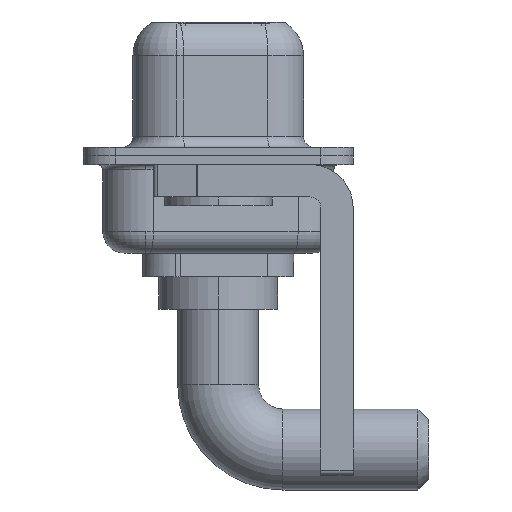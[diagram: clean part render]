
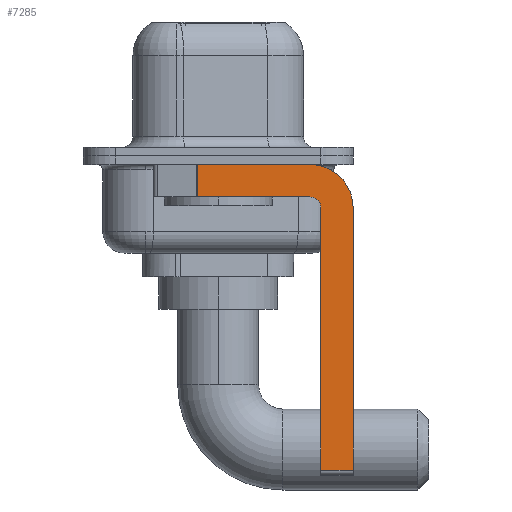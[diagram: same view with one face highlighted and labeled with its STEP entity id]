
A CAD part, left-side view. The second image highlights one B-rep face of the part: STEP entity #7285.
In plain terms, the highlighted planar face has unit normal (-1, 0, 0).
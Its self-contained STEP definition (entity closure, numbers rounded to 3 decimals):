
#55 = VERTEX_POINT ( 'NONE', #4018 ) ;
#355 = DIRECTION ( 'NONE',  ( 1., 0., 0. ) ) ;
#384 = VERTEX_POINT ( 'NONE', #9413 ) ;
#775 = LINE ( 'NONE', #13103, #7218 ) ;
#920 = ORIENTED_EDGE ( 'NONE', *, *, #1465, .F. ) ;
#1044 = CIRCLE ( 'NONE', #12889, 2. ) ;
#1110 = VECTOR ( 'NONE', #9115, 1000. ) ;
#1119 = EDGE_LOOP ( 'NONE', ( #3318, #4841, #920, #12220, #7669, #2437, #12285, #6835 ) ) ;
#1155 = EDGE_CURVE ( 'NONE', #5629, #384, #5230, .T. ) ;
#1267 = CARTESIAN_POINT ( 'NONE',  ( -2.9, -4.25, -2.4 ) ) ;
#1465 = EDGE_CURVE ( 'NONE', #8725, #384, #8699, .T. ) ;
#1575 = VERTEX_POINT ( 'NONE', #8211 ) ;
#1635 = VECTOR ( 'NONE', #11811, 1000. ) ;
#2004 = CARTESIAN_POINT ( 'NONE',  ( -2.9, -4.25, -2.4 ) ) ;
#2105 = CARTESIAN_POINT ( 'NONE',  ( -2.9, -4.75, -14.55 ) ) ;
#2138 = DIRECTION ( 'NONE',  ( 1., 0., 0. ) ) ;
#2437 = ORIENTED_EDGE ( 'NONE', *, *, #12109, .T. ) ;
#2602 = EDGE_CURVE ( 'NONE', #6748, #1575, #1044, .T. ) ;
#2878 = DIRECTION ( 'NONE',  ( -1., 0., 0. ) ) ;
#2920 = DIRECTION ( 'NONE',  ( 0., 0., 1. ) ) ;
#3006 = CARTESIAN_POINT ( 'NONE',  ( -2.9, 0.978, -1.9 ) ) ;
#3318 = ORIENTED_EDGE ( 'NONE', *, *, #8881, .F. ) ;
#3377 = CARTESIAN_POINT ( 'NONE',  ( -2.9, -4.25, -0.4 ) ) ;
#3468 = DIRECTION ( 'NONE',  ( 0., -1., 0. ) ) ;
#3838 = DIRECTION ( 'NONE',  ( 0., 1., 0. ) ) ;
#3925 = EDGE_CURVE ( 'NONE', #1575, #55, #12274, .T. ) ;
#3986 = DIRECTION ( 'NONE',  ( 0., 0., 1. ) ) ;
#4018 = CARTESIAN_POINT ( 'NONE',  ( -2.9, -6.25, -14.55 ) ) ;
#4134 = VERTEX_POINT ( 'NONE', #8537 ) ;
#4401 = DIRECTION ( 'NONE',  ( 0., 0., -1. ) ) ;
#4739 = VECTOR ( 'NONE', #3468, 1000. ) ;
#4841 = ORIENTED_EDGE ( 'NONE', *, *, #1155, .T. ) ;
#5230 = LINE ( 'NONE', #3006, #1110 ) ;
#5314 = CARTESIAN_POINT ( 'NONE',  ( -2.9, -4.25, -2.4 ) ) ;
#5629 = VERTEX_POINT ( 'NONE', #7078 ) ;
#5875 = CARTESIAN_POINT ( 'NONE',  ( -2.9, -4.25, -1.9 ) ) ;
#6292 = DIRECTION ( 'NONE',  ( 0., 0., -1. ) ) ;
#6748 = VERTEX_POINT ( 'NONE', #3377 ) ;
#6835 = ORIENTED_EDGE ( 'NONE', *, *, #2602, .F. ) ;
#7078 = CARTESIAN_POINT ( 'NONE',  ( -2.9, 0.978, -0.4 ) ) ;
#7146 = CARTESIAN_POINT ( 'NONE',  ( -2.9, -4.25, -1.9 ) ) ;
#7218 = VECTOR ( 'NONE', #2920, 1000. ) ;
#7224 = CARTESIAN_POINT ( 'NONE',  ( -2.9, -6.25, -2.4 ) ) ;
#7285 = ADVANCED_FACE ( 'NONE', ( #12128 ), #12060, .F. ) ;
#7530 = EDGE_CURVE ( 'NONE', #13018, #4134, #775, .T. ) ;
#7556 = LINE ( 'NONE', #9745, #1635 ) ;
#7669 = ORIENTED_EDGE ( 'NONE', *, *, #7530, .F. ) ;
#8211 = CARTESIAN_POINT ( 'NONE',  ( -2.9, -6.25, -2.4 ) ) ;
#8537 = CARTESIAN_POINT ( 'NONE',  ( -2.9, -4.75, -2.4 ) ) ;
#8589 = CARTESIAN_POINT ( 'NONE',  ( -2.9, 3., -0.4 ) ) ;
#8699 = LINE ( 'NONE', #5875, #9084 ) ;
#8725 = VERTEX_POINT ( 'NONE', #7146 ) ;
#8881 = EDGE_CURVE ( 'NONE', #5629, #6748, #10475, .T. ) ;
#9084 = VECTOR ( 'NONE', #3838, 1000. ) ;
#9115 = DIRECTION ( 'NONE',  ( 0., 0., -1. ) ) ;
#9413 = CARTESIAN_POINT ( 'NONE',  ( -2.9, 0.978, -1.9 ) ) ;
#9745 = CARTESIAN_POINT ( 'NONE',  ( -2.9, -4.25, -14.55 ) ) ;
#9760 = AXIS2_PLACEMENT_3D ( 'NONE', #1267, #2138, #6292 ) ;
#10089 = AXIS2_PLACEMENT_3D ( 'NONE', #2004, #2878, #3986 ) ;
#10475 = LINE ( 'NONE', #8589, #4739 ) ;
#11288 = DIRECTION ( 'NONE',  ( 0., 0., -1. ) ) ;
#11439 = VECTOR ( 'NONE', #11288, 1000. ) ;
#11811 = DIRECTION ( 'NONE',  ( 0., -1., 0. ) ) ;
#12060 = PLANE ( 'NONE',  #9760 ) ;
#12109 = EDGE_CURVE ( 'NONE', #13018, #55, #7556, .T. ) ;
#12128 = FACE_OUTER_BOUND ( 'NONE', #1119, .T. ) ;
#12220 = ORIENTED_EDGE ( 'NONE', *, *, #12742, .F. ) ;
#12274 = LINE ( 'NONE', #7224, #11439 ) ;
#12285 = ORIENTED_EDGE ( 'NONE', *, *, #3925, .F. ) ;
#12742 = EDGE_CURVE ( 'NONE', #4134, #8725, #13072, .T. ) ;
#12889 = AXIS2_PLACEMENT_3D ( 'NONE', #5314, #355, #4401 ) ;
#13018 = VERTEX_POINT ( 'NONE', #2105 ) ;
#13072 = CIRCLE ( 'NONE', #10089, 0.5 ) ;
#13103 = CARTESIAN_POINT ( 'NONE',  ( -2.9, -4.75, -14.8 ) ) ;
